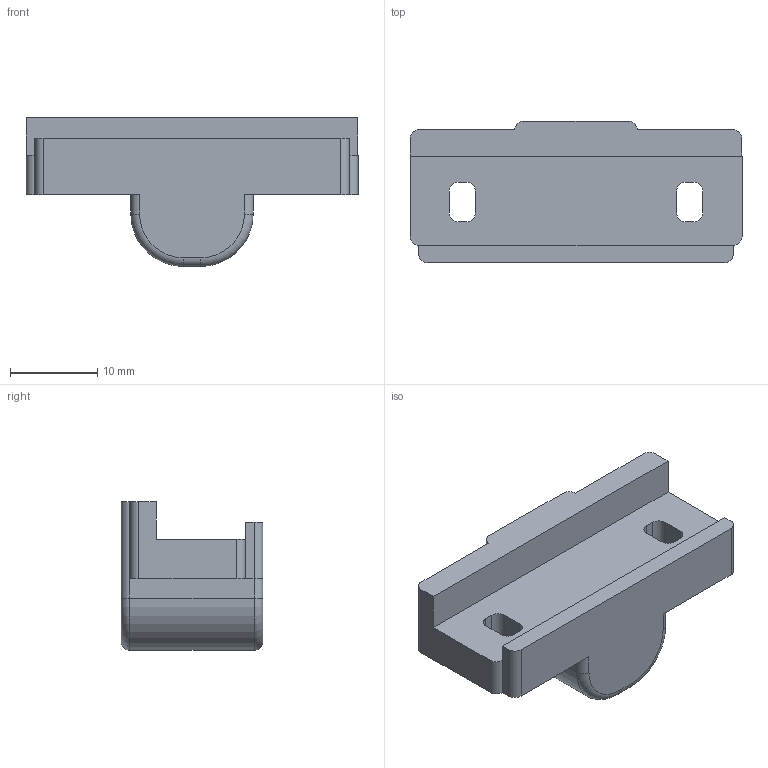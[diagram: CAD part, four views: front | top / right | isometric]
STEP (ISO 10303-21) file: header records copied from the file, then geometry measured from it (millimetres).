
FILE_DESCRIPTION (( 'STEP AP203' ), '1' );
FILE_NAME ('MOD9_ejector_mount.STEP', '2020-06-10T04:58:25', ( '' ), ( '' ), 'SwSTEP 2.0', 'SolidWorks 2016', '' );
FILE_SCHEMA (( 'CONFIG_CONTROL_DESIGN' ));
Length unit declared in the file: millimetre
Products named in the file (1): MOD9_ejector_mount
Bounding box: 38 x 16.2 x 17.04 mm (x, y, z)
Volume: 4581.2 mm3; surface area: 2794.6 mm2
Topology: 1 solids, 1 shells, 54 faces, 141 edges, 90 vertices
Faces by surface type: plane 27, cylinder 23, torus 4
Full cylindrical faces by diameter (mm): 4.4 x1
Entity records: 1739 total; most frequent: DIRECTION 300, CARTESIAN_POINT 285, ORIENTED_EDGE 280, EDGE_CURVE 140, AXIS2_PLACEMENT_3D 105, VECTOR 90, LINE 90, VERTEX_POINT 90
